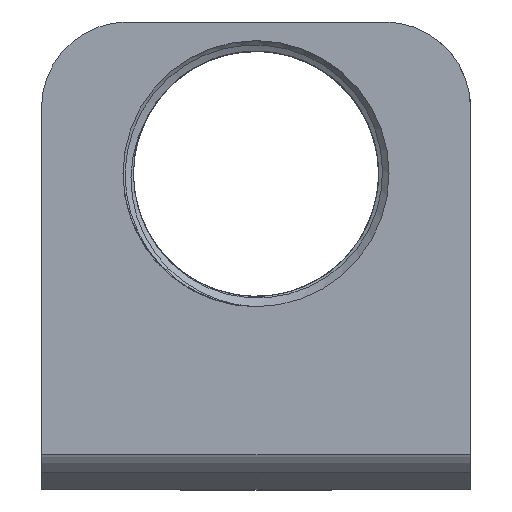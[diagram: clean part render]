
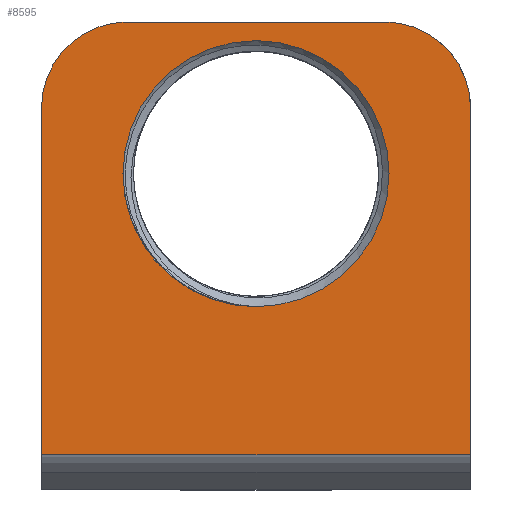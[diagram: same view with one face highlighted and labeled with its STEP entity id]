
A CAD part, top view. The second image highlights one B-rep face of the part: STEP entity #8595.
In plain terms, the highlighted planar face has unit normal (0, 0, 1).
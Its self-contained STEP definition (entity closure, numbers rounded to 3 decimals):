
#353 = CARTESIAN_POINT ( 'NONE',  ( 15., 7.678, 13.224 ) ) ;
#616 = FACE_OUTER_BOUND ( 'NONE', #2369, .T. ) ;
#1551 = CIRCLE ( 'NONE', #30914, 15.506 ) ;
#2107 = ORIENTED_EDGE ( 'NONE', *, *, #28302, .T. ) ;
#2128 = VECTOR ( 'NONE', #42232, 1000. ) ;
#2369 = EDGE_LOOP ( 'NONE', ( #17450, #39649, #29622, #2923, #2107, #31744 ) ) ;
#2607 = VECTOR ( 'NONE', #33218, 1000. ) ;
#2858 = DIRECTION ( 'NONE',  ( 0., 0., 1. ) ) ;
#2923 = ORIENTED_EDGE ( 'NONE', *, *, #15751, .T. ) ;
#3444 = VERTEX_POINT ( 'NONE', #38421 ) ;
#3706 = DIRECTION ( 'NONE',  ( 1., 0., 0. ) ) ;
#4225 = VECTOR ( 'NONE', #6664, 1000. ) ;
#6143 = VERTEX_POINT ( 'NONE', #13979 ) ;
#6664 = DIRECTION ( 'NONE',  ( -1., 0., 0. ) ) ;
#7175 = AXIS2_PLACEMENT_3D ( 'NONE', #17308, #40622, #20651 ) ;
#8558 = LINE ( 'NONE', #42205, #36183 ) ;
#8595 = ADVANCED_FACE ( 'NONE', ( #9516, #616 ), #22810, .T. ) ;
#9516 = FACE_BOUND ( 'NONE', #22177, .T. ) ;
#11133 = CARTESIAN_POINT ( 'NONE',  ( -0.03, -15.506, 13.224 ) ) ;
#11476 = LINE ( 'NONE', #29874, #2607 ) ;
#12300 = VERTEX_POINT ( 'NONE', #37930 ) ;
#13102 = LINE ( 'NONE', #29971, #4225 ) ;
#13696 = CARTESIAN_POINT ( 'NONE',  ( 0., 0., 13.224 ) ) ;
#13979 = CARTESIAN_POINT ( 'NONE',  ( -25., 7.678, 13.224 ) ) ;
#15566 = CARTESIAN_POINT ( 'NONE',  ( -25., 0., 13.224 ) ) ;
#15751 = EDGE_CURVE ( 'NONE', #3444, #40871, #13102, .T. ) ;
#16458 = EDGE_CURVE ( 'NONE', #6143, #16492, #37574, .T. ) ;
#16492 = VERTEX_POINT ( 'NONE', #28824 ) ;
#17044 = DIRECTION ( 'NONE',  ( -1., 0., 0. ) ) ;
#17308 = CARTESIAN_POINT ( 'NONE',  ( -15., 7.678, 13.224 ) ) ;
#17450 = ORIENTED_EDGE ( 'NONE', *, *, #36180, .T. ) ;
#18629 = ORIENTED_EDGE ( 'NONE', *, *, #31951, .T. ) ;
#20000 = CARTESIAN_POINT ( 'NONE',  ( 25., 7.678, 13.224 ) ) ;
#20651 = DIRECTION ( 'NONE',  ( 1., 0., 0. ) ) ;
#21047 = VERTEX_POINT ( 'NONE', #20000 ) ;
#22177 = EDGE_LOOP ( 'NONE', ( #18629 ) ) ;
#22384 = VERTEX_POINT ( 'NONE', #11133 ) ;
#22810 = PLANE ( 'NONE',  #37229 ) ;
#23252 = DIRECTION ( 'NONE',  ( 1., 0., 0. ) ) ;
#23663 = DIRECTION ( 'NONE',  ( 0., 0., 1. ) ) ;
#24664 = EDGE_CURVE ( 'NONE', #21047, #3444, #26620, .T. ) ;
#26010 = CARTESIAN_POINT ( 'NONE',  ( 0., 0., 13.224 ) ) ;
#26154 = DIRECTION ( 'NONE',  ( 1., 0., 0. ) ) ;
#26620 = CIRCLE ( 'NONE', #40935, 10. ) ;
#28302 = EDGE_CURVE ( 'NONE', #40871, #6143, #40681, .T. ) ;
#28824 = CARTESIAN_POINT ( 'NONE',  ( -25., -32.779, 13.224 ) ) ;
#29622 = ORIENTED_EDGE ( 'NONE', *, *, #24664, .T. ) ;
#29874 = CARTESIAN_POINT ( 'NONE',  ( 25., 0., 13.224 ) ) ;
#29971 = CARTESIAN_POINT ( 'NONE',  ( 0., 17.678, 13.224 ) ) ;
#30914 = AXIS2_PLACEMENT_3D ( 'NONE', #13696, #36992, #17044 ) ;
#31455 = EDGE_CURVE ( 'NONE', #12300, #21047, #11476, .T. ) ;
#31744 = ORIENTED_EDGE ( 'NONE', *, *, #16458, .T. ) ;
#31951 = EDGE_CURVE ( 'NONE', #22384, #22384, #1551, .T. ) ;
#33218 = DIRECTION ( 'NONE',  ( 0., 1., 0. ) ) ;
#36180 = EDGE_CURVE ( 'NONE', #16492, #12300, #8558, .T. ) ;
#36183 = VECTOR ( 'NONE', #23252, 1000. ) ;
#36992 = DIRECTION ( 'NONE',  ( 0., 0., -1. ) ) ;
#37068 = CARTESIAN_POINT ( 'NONE',  ( -15., 17.678, 13.224 ) ) ;
#37229 = AXIS2_PLACEMENT_3D ( 'NONE', #26010, #2858, #26154 ) ;
#37574 = LINE ( 'NONE', #15566, #2128 ) ;
#37930 = CARTESIAN_POINT ( 'NONE',  ( 25., -32.779, 13.224 ) ) ;
#38421 = CARTESIAN_POINT ( 'NONE',  ( 15., 17.678, 13.224 ) ) ;
#39649 = ORIENTED_EDGE ( 'NONE', *, *, #31455, .T. ) ;
#40622 = DIRECTION ( 'NONE',  ( 0., 0., 1. ) ) ;
#40681 = CIRCLE ( 'NONE', #7175, 10. ) ;
#40871 = VERTEX_POINT ( 'NONE', #37068 ) ;
#40935 = AXIS2_PLACEMENT_3D ( 'NONE', #353, #23663, #3706 ) ;
#42205 = CARTESIAN_POINT ( 'NONE',  ( -25., -32.779, 13.224 ) ) ;
#42232 = DIRECTION ( 'NONE',  ( 0., -1., 0. ) ) ;
